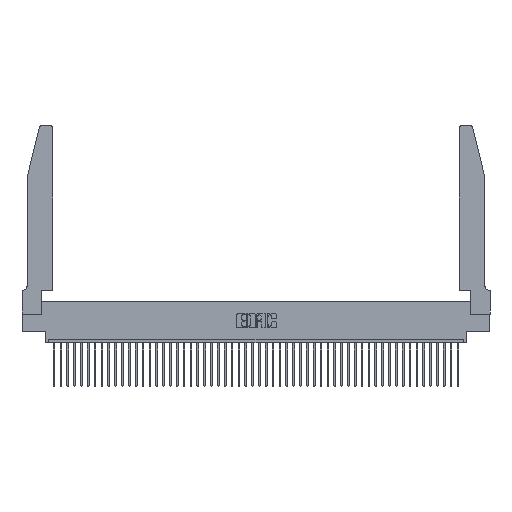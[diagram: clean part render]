
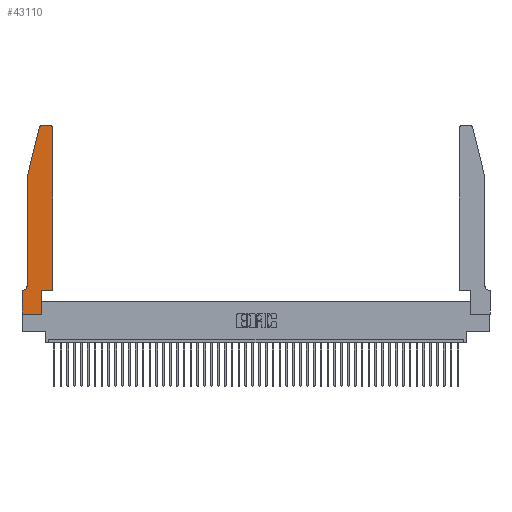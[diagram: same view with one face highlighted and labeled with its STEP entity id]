
A CAD part, top view. The second image highlights one B-rep face of the part: STEP entity #43110.
In plain terms, the highlighted planar face has unit normal (0, 0, 1).
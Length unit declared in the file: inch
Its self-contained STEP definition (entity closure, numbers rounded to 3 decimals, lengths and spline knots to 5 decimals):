
#66 = LINE ( 'NONE', #32158, #28313 ) ;
#456 = ORIENTED_EDGE ( 'NONE', *, *, #16411, .T. ) ;
#892 = AXIS2_PLACEMENT_3D ( 'NONE', #13365, #42666, #17217 ) ;
#1053 = AXIS2_PLACEMENT_3D ( 'NONE', #35978, #47172, #21458 ) ;
#1291 = FACE_OUTER_BOUND ( 'NONE', #5964, .T. ) ;
#1379 = DIRECTION ( 'NONE',  ( -0.239, -0.971, 0. ) ) ;
#3357 = CIRCLE ( 'NONE', #892, 0.03 ) ;
#4662 = VERTEX_POINT ( 'NONE', #8607 ) ;
#5362 = LINE ( 'NONE', #13939, #32411 ) ;
#5750 = CARTESIAN_POINT ( 'NONE',  ( 0.0755, 2., 0.37 ) ) ;
#5899 = VECTOR ( 'NONE', #1379, 39.37008 ) ;
#5964 = EDGE_LOOP ( 'NONE', ( #41077, #40307, #8727, #28884, #6691, #46288, #39508, #16780, #23222, #456, #47308, #29559 ) ) ;
#6225 = CARTESIAN_POINT ( 'NONE',  ( 0., 0., 0.37 ) ) ;
#6691 = ORIENTED_EDGE ( 'NONE', *, *, #10106, .T. ) ;
#8089 = DIRECTION ( 'NONE',  ( 0., 0., 1. ) ) ;
#8607 = CARTESIAN_POINT ( 'NONE',  ( 0.2865, 0., 0.37 ) ) ;
#8727 = ORIENTED_EDGE ( 'NONE', *, *, #42883, .T. ) ;
#8958 = VECTOR ( 'NONE', #33238, 39.37008 ) ;
#9373 = VERTEX_POINT ( 'NONE', #38603 ) ;
#9875 = VERTEX_POINT ( 'NONE', #30265 ) ;
#10106 = EDGE_CURVE ( 'NONE', #9875, #23211, #32542, .T. ) ;
#10797 = AXIS2_PLACEMENT_3D ( 'NONE', #42774, #46003, #27713 ) ;
#10965 = LINE ( 'NONE', #22473, #27757 ) ;
#12954 = CIRCLE ( 'NONE', #27008, 0.03 ) ;
#13183 = CARTESIAN_POINT ( 'NONE',  ( 0., 0.35, 0.37 ) ) ;
#13365 = CARTESIAN_POINT ( 'NONE',  ( 0.4205, 2.72, 0.37 ) ) ;
#13939 = CARTESIAN_POINT ( 'NONE',  ( 0., 0., 0.37 ) ) ;
#14017 = VERTEX_POINT ( 'NONE', #23866 ) ;
#14566 = VECTOR ( 'NONE', #16658, 39.37008 ) ;
#15158 = CARTESIAN_POINT ( 'NONE',  ( 0.0055, 0.35, 0.37 ) ) ;
#15211 = VERTEX_POINT ( 'NONE', #42892 ) ;
#15957 = CARTESIAN_POINT ( 'NONE',  ( 0.0755, 2., 0.37 ) ) ;
#16411 = EDGE_CURVE ( 'NONE', #17712, #37077, #66, .T. ) ;
#16658 = DIRECTION ( 'NONE',  ( 0., -1., 0. ) ) ;
#16780 = ORIENTED_EDGE ( 'NONE', *, *, #20150, .T. ) ;
#17217 = DIRECTION ( 'NONE',  ( 1., 0., 0. ) ) ;
#17712 = VERTEX_POINT ( 'NONE', #28482 ) ;
#17715 = PLANE ( 'NONE',  #1053 ) ;
#18415 = CARTESIAN_POINT ( 'NONE',  ( 0.2605, 2.75, 0.37 ) ) ;
#18541 = CARTESIAN_POINT ( 'NONE',  ( 0., 0., 0.37 ) ) ;
#20150 = EDGE_CURVE ( 'NONE', #36677, #4662, #32148, .T. ) ;
#20970 = VECTOR ( 'NONE', #22605, 39.37008 ) ;
#21458 = DIRECTION ( 'NONE',  ( 1., 0., 0. ) ) ;
#21671 = EDGE_CURVE ( 'NONE', #37077, #15211, #37731, .T. ) ;
#21856 = CARTESIAN_POINT ( 'NONE',  ( 0.4505, 0.35, 0.37 ) ) ;
#22099 = CARTESIAN_POINT ( 'NONE',  ( 0.0755, 0.35, 0.37 ) ) ;
#22373 = EDGE_CURVE ( 'NONE', #9373, #25082, #28491, .T. ) ;
#22473 = CARTESIAN_POINT ( 'NONE',  ( 0.2865, 0.35, 0.37 ) ) ;
#22605 = DIRECTION ( 'NONE',  ( -1., 0., 0. ) ) ;
#23211 = VERTEX_POINT ( 'NONE', #15158 ) ;
#23222 = ORIENTED_EDGE ( 'NONE', *, *, #29434, .T. ) ;
#23357 = EDGE_CURVE ( 'NONE', #14017, #9875, #47412, .T. ) ;
#23866 = CARTESIAN_POINT ( 'NONE',  ( 0.0755, 2., 0.37 ) ) ;
#24376 = DIRECTION ( 'NONE',  ( 0., 1., 0. ) ) ;
#24680 = VECTOR ( 'NONE', #42899, 39.37008 ) ;
#25082 = VERTEX_POINT ( 'NONE', #40942 ) ;
#26223 = DIRECTION ( 'NONE',  ( 0., 1., 0. ) ) ;
#27008 = AXIS2_PLACEMENT_3D ( 'NONE', #44452, #8089, #30319 ) ;
#27028 = EDGE_CURVE ( 'NONE', #23211, #38437, #31407, .T. ) ;
#27048 = EDGE_CURVE ( 'NONE', #25082, #43254, #12954, .T. ) ;
#27713 = DIRECTION ( 'NONE',  ( -1., 0., 0. ) ) ;
#27757 = VECTOR ( 'NONE', #26223, 39.37008 ) ;
#28313 = VECTOR ( 'NONE', #43553, 39.37008 ) ;
#28482 = CARTESIAN_POINT ( 'NONE',  ( 0.2865, 0.35, 0.37 ) ) ;
#28491 = LINE ( 'NONE', #18415, #20970 ) ;
#28650 = DIRECTION ( 'NONE',  ( 0., -1., 0. ) ) ;
#28659 = EDGE_CURVE ( 'NONE', #38437, #36677, #5362, .T. ) ;
#28884 = ORIENTED_EDGE ( 'NONE', *, *, #23357, .T. ) ;
#29434 = EDGE_CURVE ( 'NONE', #4662, #17712, #10965, .T. ) ;
#29559 = ORIENTED_EDGE ( 'NONE', *, *, #31219, .T. ) ;
#30265 = CARTESIAN_POINT ( 'NONE',  ( 0.0755, 0.42, 0.37 ) ) ;
#30319 = DIRECTION ( 'NONE',  ( 1., 0., 0. ) ) ;
#31219 = EDGE_CURVE ( 'NONE', #15211, #9373, #3357, .T. ) ;
#31407 = LINE ( 'NONE', #22099, #8958 ) ;
#32148 = LINE ( 'NONE', #6225, #24680 ) ;
#32158 = CARTESIAN_POINT ( 'NONE',  ( 0.4505, 0.35, 0.37 ) ) ;
#32411 = VECTOR ( 'NONE', #28650, 39.37008 ) ;
#32542 = CIRCLE ( 'NONE', #10797, 0.07 ) ;
#32979 = LINE ( 'NONE', #15957, #5899 ) ;
#33238 = DIRECTION ( 'NONE',  ( -1., 0., 0. ) ) ;
#33723 = VECTOR ( 'NONE', #24376, 39.37008 ) ;
#35978 = CARTESIAN_POINT ( 'NONE',  ( 0., 0.35, 0.37 ) ) ;
#36677 = VERTEX_POINT ( 'NONE', #18541 ) ;
#37077 = VERTEX_POINT ( 'NONE', #21856 ) ;
#37707 = CARTESIAN_POINT ( 'NONE',  ( 0.25487, 2.72718, 0.37 ) ) ;
#37731 = LINE ( 'NONE', #46568, #33723 ) ;
#38437 = VERTEX_POINT ( 'NONE', #13183 ) ;
#38603 = CARTESIAN_POINT ( 'NONE',  ( 0.4205, 2.75, 0.37 ) ) ;
#39508 = ORIENTED_EDGE ( 'NONE', *, *, #28659, .T. ) ;
#40307 = ORIENTED_EDGE ( 'NONE', *, *, #27048, .T. ) ;
#40942 = CARTESIAN_POINT ( 'NONE',  ( 0.284, 2.75, 0.37 ) ) ;
#41077 = ORIENTED_EDGE ( 'NONE', *, *, #22373, .T. ) ;
#42666 = DIRECTION ( 'NONE',  ( 0., 0., 1. ) ) ;
#42774 = CARTESIAN_POINT ( 'NONE',  ( 0.0055, 0.42, 0.37 ) ) ;
#42883 = EDGE_CURVE ( 'NONE', #43254, #14017, #32979, .T. ) ;
#42892 = CARTESIAN_POINT ( 'NONE',  ( 0.4505, 2.72, 0.37 ) ) ;
#42899 = DIRECTION ( 'NONE',  ( 1., 0., 0. ) ) ;
#43110 = ADVANCED_FACE ( 'NONE', ( #1291 ), #17715, .T. ) ;
#43254 = VERTEX_POINT ( 'NONE', #37707 ) ;
#43553 = DIRECTION ( 'NONE',  ( 1., 0., 0. ) ) ;
#44452 = CARTESIAN_POINT ( 'NONE',  ( 0.284, 2.72, 0.37 ) ) ;
#46003 = DIRECTION ( 'NONE',  ( 0., 0., -1. ) ) ;
#46288 = ORIENTED_EDGE ( 'NONE', *, *, #27028, .T. ) ;
#46568 = CARTESIAN_POINT ( 'NONE',  ( 0.4505, 0.35, 0.37 ) ) ;
#47172 = DIRECTION ( 'NONE',  ( 0., 0., 1. ) ) ;
#47308 = ORIENTED_EDGE ( 'NONE', *, *, #21671, .T. ) ;
#47412 = LINE ( 'NONE', #5750, #14566 ) ;
